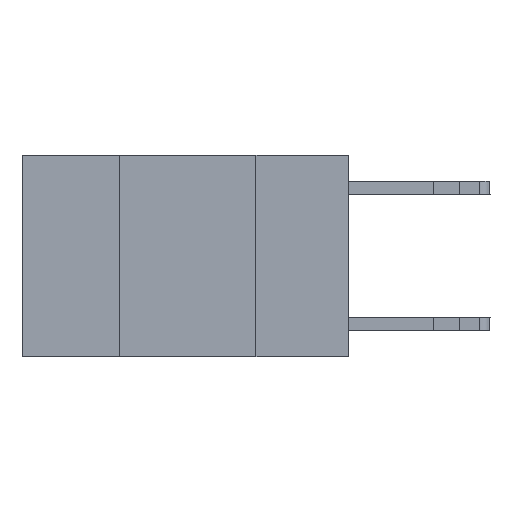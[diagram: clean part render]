
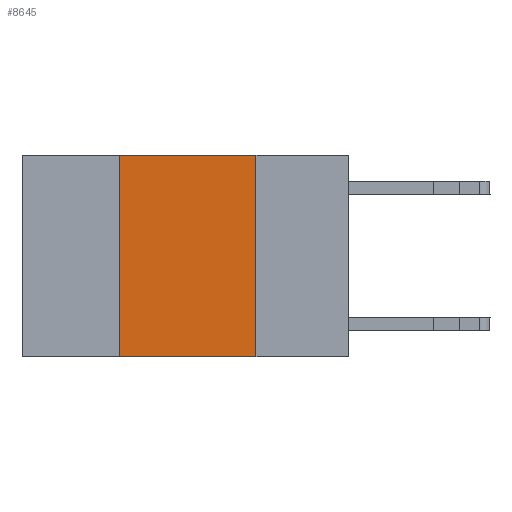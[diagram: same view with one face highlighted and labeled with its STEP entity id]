
A CAD part, left-side view. The second image highlights one B-rep face of the part: STEP entity #8645.
In plain terms, the highlighted planar face has unit normal (-1, 0, 0).
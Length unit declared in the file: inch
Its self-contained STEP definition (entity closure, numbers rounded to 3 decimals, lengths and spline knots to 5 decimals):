
#11 = EDGE_CURVE ( 'NONE', #2498, #4355, #11350, .T. ) ;
#410 = DIRECTION ( 'NONE',  ( 0., 0., -1. ) ) ;
#498 = LINE ( 'NONE', #6449, #3058 ) ;
#570 = DIRECTION ( 'NONE',  ( 1., 0., 0. ) ) ;
#919 = DIRECTION ( 'NONE',  ( 0., 0., 1. ) ) ;
#1048 = EDGE_CURVE ( 'NONE', #2498, #6475, #9523, .T. ) ;
#1057 = EDGE_LOOP ( 'NONE', ( #10625, #9102, #12259, #11894 ) ) ;
#1142 = DIRECTION ( 'NONE',  ( 0., -1., 0. ) ) ;
#1357 = LINE ( 'NONE', #9003, #7479 ) ;
#1389 = AXIS2_PLACEMENT_3D ( 'NONE', #2488, #570, #8343 ) ;
#1516 = PLANE ( 'NONE',  #1389 ) ;
#2197 = EDGE_CURVE ( 'NONE', #4355, #10659, #498, .T. ) ;
#2488 = CARTESIAN_POINT ( 'NONE',  ( 0., 0.6, 0. ) ) ;
#2498 = VERTEX_POINT ( 'NONE', #11298 ) ;
#3058 = VECTOR ( 'NONE', #4587, 39.37008 ) ;
#3436 = FACE_OUTER_BOUND ( 'NONE', #1057, .T. ) ;
#3576 = VECTOR ( 'NONE', #919, 39.37008 ) ;
#4355 = VERTEX_POINT ( 'NONE', #11697 ) ;
#4587 = DIRECTION ( 'NONE',  ( 0., -1., 0. ) ) ;
#4918 = CARTESIAN_POINT ( 'NONE',  ( 0., 0.6, -0.37 ) ) ;
#5965 = CARTESIAN_POINT ( 'NONE',  ( 0., 0.17, 0. ) ) ;
#6449 = CARTESIAN_POINT ( 'NONE',  ( 0., 0.6, 0. ) ) ;
#6475 = VERTEX_POINT ( 'NONE', #10655 ) ;
#7479 = VECTOR ( 'NONE', #410, 39.37008 ) ;
#8343 = DIRECTION ( 'NONE',  ( 0., 0., -1. ) ) ;
#8645 = ADVANCED_FACE ( 'NONE', ( #3436 ), #1516, .F. ) ;
#9003 = CARTESIAN_POINT ( 'NONE',  ( 0., 0.17, 0. ) ) ;
#9102 = ORIENTED_EDGE ( 'NONE', *, *, #2197, .F. ) ;
#9418 = VECTOR ( 'NONE', #1142, 39.37008 ) ;
#9523 = LINE ( 'NONE', #4918, #9418 ) ;
#10625 = ORIENTED_EDGE ( 'NONE', *, *, #11940, .F. ) ;
#10655 = CARTESIAN_POINT ( 'NONE',  ( 0., 0.17, -0.37 ) ) ;
#10659 = VERTEX_POINT ( 'NONE', #5965 ) ;
#11298 = CARTESIAN_POINT ( 'NONE',  ( 0., 0.42, -0.37 ) ) ;
#11350 = LINE ( 'NONE', #12318, #3576 ) ;
#11697 = CARTESIAN_POINT ( 'NONE',  ( 0., 0.42, 0. ) ) ;
#11894 = ORIENTED_EDGE ( 'NONE', *, *, #1048, .T. ) ;
#11940 = EDGE_CURVE ( 'NONE', #10659, #6475, #1357, .T. ) ;
#12259 = ORIENTED_EDGE ( 'NONE', *, *, #11, .F. ) ;
#12318 = CARTESIAN_POINT ( 'NONE',  ( 0., 0.42, 0. ) ) ;
